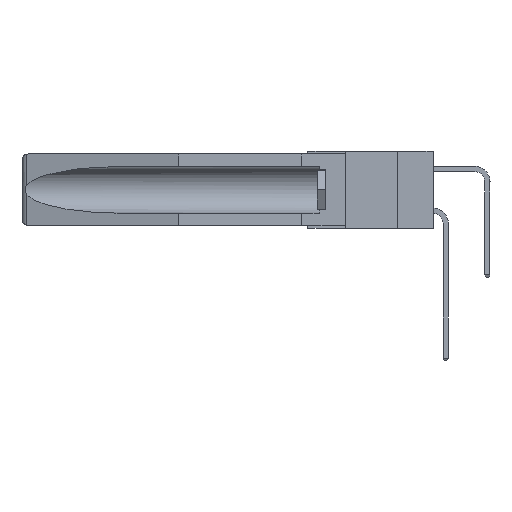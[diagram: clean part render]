
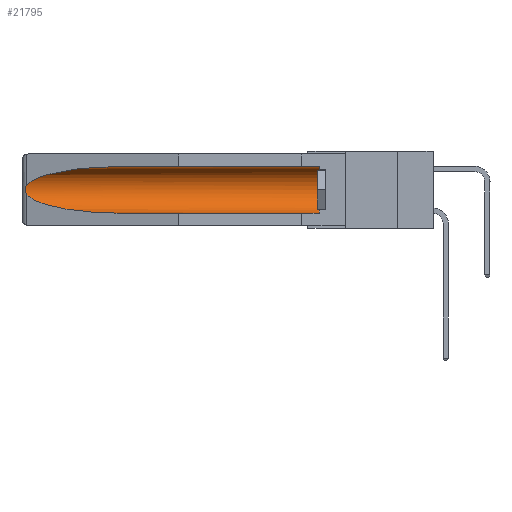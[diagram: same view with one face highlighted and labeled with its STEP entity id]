
A CAD part, left-side view. The second image highlights one B-rep face of the part: STEP entity #21795.
In plain terms, the highlighted cylindrical face has radius 2.857 mm (diameter 5.715 mm), a partial arc.
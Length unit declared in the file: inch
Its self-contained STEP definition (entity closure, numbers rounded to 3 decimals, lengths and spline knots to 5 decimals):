
#577 = ORIENTED_EDGE ( 'NONE', *, *, #19299, .T. ) ;
#907 = B_SPLINE_CURVE_WITH_KNOTS ( 'NONE', 3,
 ( #10468, #4943, #16376, #4694, #22295, #18592, #10551, #8827, #16460, #4779 ),
 .UNSPECIFIED., .F., .F.,
 ( 4, 2, 2, 2, 4 ),
 ( 0., 0.00029, 0.00058, 0.00087, 0.00117 ),
 .UNSPECIFIED. ) ;
#1161 = FACE_OUTER_BOUND ( 'NONE', #17985, .T. ) ;
#1352 = VERTEX_POINT ( 'NONE', #2054 ) ;
#1593 = CARTESIAN_POINT ( 'NONE',  ( 0.155, 0.126, -0.059 ) ) ;
#2054 = CARTESIAN_POINT ( 'NONE',  ( 0.155, 0.126, -0.284 ) ) ;
#2420 = ORIENTED_EDGE ( 'NONE', *, *, #12466, .T. ) ;
#3010 = ORIENTED_EDGE ( 'NONE', *, *, #18025, .T. ) ;
#3595 = CIRCLE ( 'NONE', #8069, 0.1125 ) ;
#4182 =( BOUNDED_CURVE ( )  B_SPLINE_CURVE ( 3, ( #16267, #8488, #12747, #20592 ),
 .UNSPECIFIED., .F., .F. ) 
 B_SPLINE_CURVE_WITH_KNOTS ( ( 4, 4 ),
 ( 0.1948, 1.5708 ),
 .UNSPECIFIED. ) 
 CURVE ( )  GEOMETRIC_REPRESENTATION_ITEM ( )  RATIONAL_B_SPLINE_CURVE ( ( 1., 0.848, 0.848, 1. ) ) 
 REPRESENTATION_ITEM ( '' )  );
#4294 = CARTESIAN_POINT ( 'NONE',  ( 0.26537, 1.52718, -0.14972 ) ) ;
#4694 = CARTESIAN_POINT ( 'NONE',  ( 0.2673, 1.5327, -0.16383 ) ) ;
#4779 = CARTESIAN_POINT ( 'NONE',  ( 0.26537, 1.52718, -0.19328 ) ) ;
#4835 = AXIS2_PLACEMENT_3D ( 'NONE', #11062, #20849, #17069 ) ;
#4943 = CARTESIAN_POINT ( 'NONE',  ( 0.26597, 1.52961, -0.15275 ) ) ;
#5010 = DIRECTION ( 'NONE',  ( 0., -1., 0. ) ) ;
#5502 = ORIENTED_EDGE ( 'NONE', *, *, #20616, .F. ) ;
#5579 = VERTEX_POINT ( 'NONE', #1593 ) ;
#5693 = CYLINDRICAL_SURFACE ( 'NONE', #4835, 0.1125 ) ;
#7000 = LINE ( 'NONE', #14716, #19233 ) ;
#8050 = VERTEX_POINT ( 'NONE', #9851 ) ;
#8069 = AXIS2_PLACEMENT_3D ( 'NONE', #16706, #5010, #11129 ) ;
#8428 = ORIENTED_EDGE ( 'NONE', *, *, #10178, .T. ) ;
#8488 = CARTESIAN_POINT ( 'NONE',  ( 0.25451, 1.48313, -0.24835 ) ) ;
#8599 = CARTESIAN_POINT ( 'NONE',  ( 0.155, 1.07973, -0.059 ) ) ;
#8649 = ORIENTED_EDGE ( 'NONE', *, *, #22808, .T. ) ;
#8827 = CARTESIAN_POINT ( 'NONE',  ( 0.26655, 1.53094, -0.18657 ) ) ;
#9851 = CARTESIAN_POINT ( 'NONE',  ( 0.155, 1.07973, -0.284 ) ) ;
#9890 = CARTESIAN_POINT ( 'NONE',  ( 0.25451, 1.48313, -0.09465 ) ) ;
#10075 = VERTEX_POINT ( 'NONE', #8599 ) ;
#10178 = EDGE_CURVE ( 'NONE', #1352, #5579, #3595, .T. ) ;
#10468 = CARTESIAN_POINT ( 'NONE',  ( 0.26537, 1.52718, -0.14972 ) ) ;
#10551 = CARTESIAN_POINT ( 'NONE',  ( 0.2673, 1.53269, -0.17917 ) ) ;
#11062 = CARTESIAN_POINT ( 'NONE',  ( 0.155, -0.30754, -0.1715 ) ) ;
#11129 = DIRECTION ( 'NONE',  ( 0., 0., 1. ) ) ;
#12466 = EDGE_CURVE ( 'NONE', #10075, #21709, #15916, .T. ) ;
#12747 = CARTESIAN_POINT ( 'NONE',  ( 0.21114, 1.30732, -0.284 ) ) ;
#14716 = CARTESIAN_POINT ( 'NONE',  ( 0.155, -0.30754, -0.284 ) ) ;
#15916 =( BOUNDED_CURVE ( )  B_SPLINE_CURVE ( 3, ( #23770, #23856, #9890, #4294 ),
 .UNSPECIFIED., .F., .F. ) 
 B_SPLINE_CURVE_WITH_KNOTS ( ( 4, 4 ),
 ( 4.71239, 6.08839 ),
 .UNSPECIFIED. ) 
 CURVE ( )  GEOMETRIC_REPRESENTATION_ITEM ( )  RATIONAL_B_SPLINE_CURVE ( ( 1., 0.848, 0.848, 1. ) ) 
 REPRESENTATION_ITEM ( '' )  );
#15930 = LINE ( 'NONE', #18744, #20242 ) ;
#16267 = CARTESIAN_POINT ( 'NONE',  ( 0.26537, 1.52718, -0.19328 ) ) ;
#16376 = CARTESIAN_POINT ( 'NONE',  ( 0.26654, 1.53092, -0.15636 ) ) ;
#16460 = CARTESIAN_POINT ( 'NONE',  ( 0.26597, 1.5296, -0.19026 ) ) ;
#16706 = CARTESIAN_POINT ( 'NONE',  ( 0.155, 0.126, -0.1715 ) ) ;
#17069 = DIRECTION ( 'NONE',  ( 0., 0., 1. ) ) ;
#17985 = EDGE_LOOP ( 'NONE', ( #2420, #3010, #8649, #5502, #8428, #577 ) ) ;
#18025 = EDGE_CURVE ( 'NONE', #21709, #22076, #907, .T. ) ;
#18592 = CARTESIAN_POINT ( 'NONE',  ( 0.2675, 1.53308, -0.17534 ) ) ;
#18744 = CARTESIAN_POINT ( 'NONE',  ( 0.155, -0.30754, -0.059 ) ) ;
#19233 = VECTOR ( 'NONE', #24774, 39.37008 ) ;
#19299 = EDGE_CURVE ( 'NONE', #5579, #10075, #15930, .T. ) ;
#20242 = VECTOR ( 'NONE', #22619, 39.37008 ) ;
#20592 = CARTESIAN_POINT ( 'NONE',  ( 0.155, 1.07973, -0.284 ) ) ;
#20616 = EDGE_CURVE ( 'NONE', #1352, #8050, #7000, .T. ) ;
#20849 = DIRECTION ( 'NONE',  ( 0., 1., 0. ) ) ;
#21519 = CARTESIAN_POINT ( 'NONE',  ( 0.26537, 1.52718, -0.19328 ) ) ;
#21709 = VERTEX_POINT ( 'NONE', #23854 ) ;
#21795 = ADVANCED_FACE ( 'NONE', ( #1161 ), #5693, .F. ) ;
#22076 = VERTEX_POINT ( 'NONE', #21519 ) ;
#22295 = CARTESIAN_POINT ( 'NONE',  ( 0.2675, 1.53308, -0.16763 ) ) ;
#22619 = DIRECTION ( 'NONE',  ( 0., 1., 0. ) ) ;
#22808 = EDGE_CURVE ( 'NONE', #22076, #8050, #4182, .T. ) ;
#23770 = CARTESIAN_POINT ( 'NONE',  ( 0.155, 1.07973, -0.059 ) ) ;
#23854 = CARTESIAN_POINT ( 'NONE',  ( 0.26537, 1.52718, -0.14972 ) ) ;
#23856 = CARTESIAN_POINT ( 'NONE',  ( 0.21114, 1.30732, -0.059 ) ) ;
#24774 = DIRECTION ( 'NONE',  ( 0., 1., 0. ) ) ;
